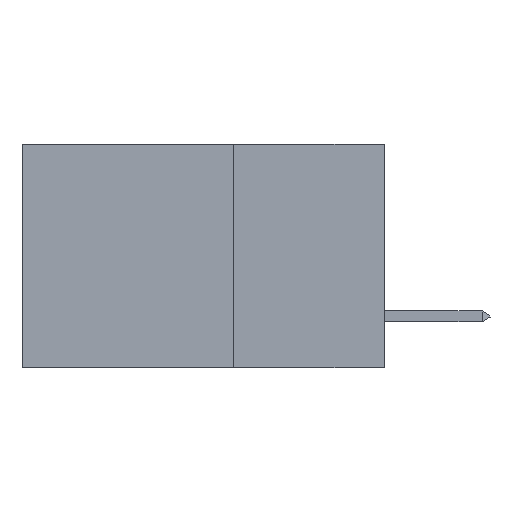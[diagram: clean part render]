
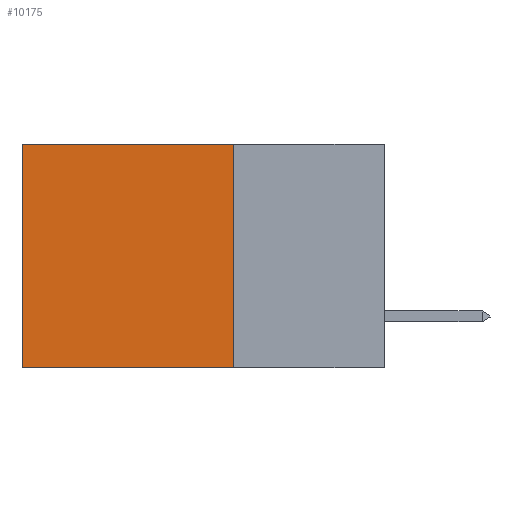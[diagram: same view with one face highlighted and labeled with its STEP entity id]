
A CAD part, left-side view. The second image highlights one B-rep face of the part: STEP entity #10175.
In plain terms, the highlighted planar face has unit normal (-1, 0, 0).
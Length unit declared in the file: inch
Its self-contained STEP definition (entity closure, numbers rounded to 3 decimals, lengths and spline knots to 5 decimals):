
#14 = VERTEX_POINT ( 'NONE', #8290 ) ;
#447 = CARTESIAN_POINT ( 'NONE',  ( 0.2875, 0.25, 0. ) ) ;
#457 = DIRECTION ( 'NONE',  ( 0., 0., -1. ) ) ;
#557 = CARTESIAN_POINT ( 'NONE',  ( 0.2875, 0.25, 0. ) ) ;
#1589 = VERTEX_POINT ( 'NONE', #8951 ) ;
#1756 = VERTEX_POINT ( 'NONE', #14085 ) ;
#1771 = CARTESIAN_POINT ( 'NONE',  ( 0.2875, 0.6, 0. ) ) ;
#1874 = CARTESIAN_POINT ( 'NONE',  ( 0.2875, 0.25, -0.37 ) ) ;
#1881 = EDGE_CURVE ( 'NONE', #4384, #1589, #4264, .T. ) ;
#2329 = EDGE_LOOP ( 'NONE', ( #7594, #3286, #10243, #15111 ) ) ;
#2345 = VECTOR ( 'NONE', #13129, 39.37008 ) ;
#3286 = ORIENTED_EDGE ( 'NONE', *, *, #15014, .F. ) ;
#3377 = EDGE_CURVE ( 'NONE', #14, #4384, #9057, .T. ) ;
#4195 = PLANE ( 'NONE',  #12508 ) ;
#4264 = LINE ( 'NONE', #16147, #15284 ) ;
#4384 = VERTEX_POINT ( 'NONE', #1771 ) ;
#4680 = VECTOR ( 'NONE', #11909, 39.37008 ) ;
#4886 = DIRECTION ( 'NONE',  ( 0., 0., -1. ) ) ;
#5049 = CARTESIAN_POINT ( 'NONE',  ( 0.2875, 0.25, 0. ) ) ;
#5148 = DIRECTION ( 'NONE',  ( 0., 0., -1. ) ) ;
#6718 = LINE ( 'NONE', #5049, #11018 ) ;
#6746 = FACE_OUTER_BOUND ( 'NONE', #2329, .T. ) ;
#7594 = ORIENTED_EDGE ( 'NONE', *, *, #1881, .T. ) ;
#8290 = CARTESIAN_POINT ( 'NONE',  ( 0.2875, 0.25, 0. ) ) ;
#8951 = CARTESIAN_POINT ( 'NONE',  ( 0.2875, 0.6, -0.37 ) ) ;
#9057 = LINE ( 'NONE', #447, #2345 ) ;
#10175 = ADVANCED_FACE ( 'NONE', ( #6746 ), #4195, .F. ) ;
#10243 = ORIENTED_EDGE ( 'NONE', *, *, #11335, .F. ) ;
#11018 = VECTOR ( 'NONE', #5148, 39.37008 ) ;
#11335 = EDGE_CURVE ( 'NONE', #14, #1756, #6718, .T. ) ;
#11909 = DIRECTION ( 'NONE',  ( 0., 1., 0. ) ) ;
#12508 = AXIS2_PLACEMENT_3D ( 'NONE', #557, #13196, #457 ) ;
#13129 = DIRECTION ( 'NONE',  ( 0., 1., 0. ) ) ;
#13196 = DIRECTION ( 'NONE',  ( 1., 0., 0. ) ) ;
#14085 = CARTESIAN_POINT ( 'NONE',  ( 0.2875, 0.25, -0.37 ) ) ;
#15014 = EDGE_CURVE ( 'NONE', #1756, #1589, #15899, .T. ) ;
#15111 = ORIENTED_EDGE ( 'NONE', *, *, #3377, .T. ) ;
#15284 = VECTOR ( 'NONE', #4886, 39.37008 ) ;
#15899 = LINE ( 'NONE', #1874, #4680 ) ;
#16147 = CARTESIAN_POINT ( 'NONE',  ( 0.2875, 0.6, 0. ) ) ;
